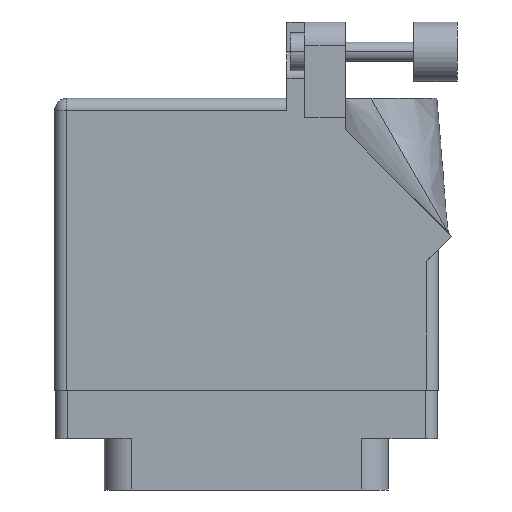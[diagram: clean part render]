
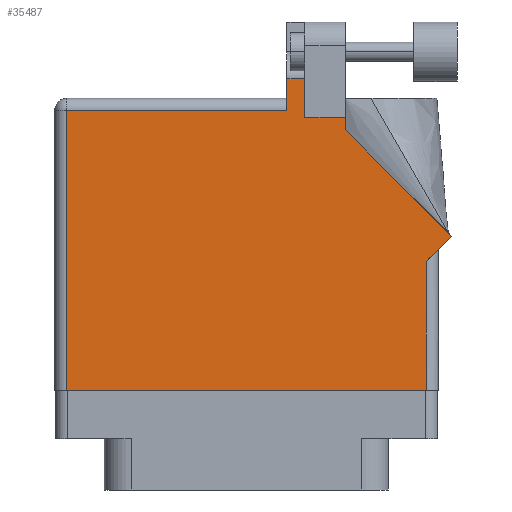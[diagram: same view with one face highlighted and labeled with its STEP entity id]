
A CAD part, front view. The second image highlights one B-rep face of the part: STEP entity #35487.
In plain terms, the highlighted face is planar.
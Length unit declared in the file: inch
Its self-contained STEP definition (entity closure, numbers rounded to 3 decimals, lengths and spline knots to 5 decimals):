
#379 = VECTOR ( 'NONE', #23614, 39.37008 ) ;
#653 = VECTOR ( 'NONE', #24554, 39.37008 ) ;
#1255 = EDGE_CURVE ( 'NONE', #32799, #14136, #2132, .T. ) ;
#1619 = ORIENTED_EDGE ( 'NONE', *, *, #6178, .T. ) ;
#2132 = LINE ( 'NONE', #20921, #379 ) ;
#3092 = ORIENTED_EDGE ( 'NONE', *, *, #34609, .T. ) ;
#3384 = VERTEX_POINT ( 'NONE', #27322 ) ;
#3631 = VECTOR ( 'NONE', #16122, 39.37008 ) ;
#3698 = AXIS2_PLACEMENT_3D ( 'NONE', #28325, #28918, #32117 ) ;
#4197 = CARTESIAN_POINT ( 'NONE',  ( 0.306, 1.33, 0.455 ) ) ;
#4200 = LINE ( 'NONE', #22063, #33316 ) ;
#4429 = LINE ( 'NONE', #13375, #14575 ) ;
#5125 = CARTESIAN_POINT ( 'NONE',  ( 0.63677, 1.5315, 0.455 ) ) ;
#6178 = EDGE_CURVE ( 'NONE', #30503, #13214, #19318, .T. ) ;
#6745 = ORIENTED_EDGE ( 'NONE', *, *, #1255, .T. ) ;
#7783 = DIRECTION ( 'NONE',  ( -0.707, 0.707, 0. ) ) ;
#8023 = CARTESIAN_POINT ( 'NONE',  ( 0.519, 1.26442, 0.455 ) ) ;
#8145 = LINE ( 'NONE', #21734, #653 ) ;
#8902 = ORIENTED_EDGE ( 'NONE', *, *, #35794, .T. ) ;
#9050 = CARTESIAN_POINT ( 'NONE',  ( -0.943, -0.1, 0.455 ) ) ;
#9063 = LINE ( 'NONE', #27660, #13047 ) ;
#9408 = CARTESIAN_POINT ( 'NONE',  ( 1.07571, 0.70771, 0.455 ) ) ;
#10152 = EDGE_CURVE ( 'NONE', #3384, #30298, #11597, .T. ) ;
#10605 = CARTESIAN_POINT ( 'NONE',  ( 0.519, 1.26442, 0.455 ) ) ;
#11462 = VECTOR ( 'NONE', #28181, 39.37008 ) ;
#11514 = ORIENTED_EDGE ( 'NONE', *, *, #27716, .T. ) ;
#11526 = VECTOR ( 'NONE', #19142, 39.37008 ) ;
#11597 = LINE ( 'NONE', #21714, #3631 ) ;
#12305 = VERTEX_POINT ( 'NONE', #13595 ) ;
#12872 = DIRECTION ( 'NONE',  ( 0., -1., 0. ) ) ;
#13047 = VECTOR ( 'NONE', #36374, 39.37008 ) ;
#13214 = VERTEX_POINT ( 'NONE', #8023 ) ;
#13375 = CARTESIAN_POINT ( 'NONE',  ( 1.005, 0.637, 0.455 ) ) ;
#13595 = CARTESIAN_POINT ( 'NONE',  ( 0.306, 1.5315, 0.455 ) ) ;
#14136 = VERTEX_POINT ( 'NONE', #34567 ) ;
#14575 = VECTOR ( 'NONE', #16202, 39.37008 ) ;
#14592 = VECTOR ( 'NONE', #23226, 39.37008 ) ;
#15504 = LINE ( 'NONE', #10605, #11526 ) ;
#15553 = ORIENTED_EDGE ( 'NONE', *, *, #17879, .T. ) ;
#16122 = DIRECTION ( 'NONE',  ( 0., -1., 0. ) ) ;
#16136 = VECTOR ( 'NONE', #12872, 39.37008 ) ;
#16202 = DIRECTION ( 'NONE',  ( 0.707, 0.707, 0. ) ) ;
#16537 = VERTEX_POINT ( 'NONE', #33179 ) ;
#17108 = VECTOR ( 'NONE', #7783, 39.37008 ) ;
#17392 = VERTEX_POINT ( 'NONE', #18812 ) ;
#17879 = EDGE_CURVE ( 'NONE', #33419, #17392, #23655, .T. ) ;
#18084 = FACE_OUTER_BOUND ( 'NONE', #23627, .T. ) ;
#18812 = CARTESIAN_POINT ( 'NONE',  ( 0.212, 1.368, 0.455 ) ) ;
#19142 = DIRECTION ( 'NONE',  ( 0., 1., 0. ) ) ;
#19318 = LINE ( 'NONE', #36235, #17108 ) ;
#19825 = PLANE ( 'NONE',  #3698 ) ;
#20921 = CARTESIAN_POINT ( 'NONE',  ( 0.943, 0.637, 0.455 ) ) ;
#20997 = VERTEX_POINT ( 'NONE', #4197 ) ;
#21714 = CARTESIAN_POINT ( 'NONE',  ( -0.943, -0.1, 0.455 ) ) ;
#21734 = CARTESIAN_POINT ( 'NONE',  ( -1.005, -0.1, 0.455 ) ) ;
#22063 = CARTESIAN_POINT ( 'NONE',  ( 0.519, 1.33, 0.455 ) ) ;
#22967 = LINE ( 'NONE', #23095, #14592 ) ;
#23095 = CARTESIAN_POINT ( 'NONE',  ( 0.306, 1.33, 0.455 ) ) ;
#23226 = DIRECTION ( 'NONE',  ( 0., 1., 0. ) ) ;
#23614 = DIRECTION ( 'NONE',  ( 0., 1., 0. ) ) ;
#23627 = EDGE_LOOP ( 'NONE', ( #33123, #8902, #15553, #27312, #23972, #25921, #6745, #32925, #1619, #3092, #11514 ) ) ;
#23655 = LINE ( 'NONE', #29771, #16136 ) ;
#23972 = ORIENTED_EDGE ( 'NONE', *, *, #10152, .T. ) ;
#24507 = EDGE_CURVE ( 'NONE', #14136, #30503, #4429, .T. ) ;
#24554 = DIRECTION ( 'NONE',  ( 1., 0., 0. ) ) ;
#25921 = ORIENTED_EDGE ( 'NONE', *, *, #31208, .T. ) ;
#27004 = EDGE_CURVE ( 'NONE', #17392, #3384, #9063, .T. ) ;
#27312 = ORIENTED_EDGE ( 'NONE', *, *, #27004, .T. ) ;
#27322 = CARTESIAN_POINT ( 'NONE',  ( -0.943, 1.368, 0.455 ) ) ;
#27660 = CARTESIAN_POINT ( 'NONE',  ( -1.005, 1.368, 0.455 ) ) ;
#27716 = EDGE_CURVE ( 'NONE', #16537, #20997, #4200, .T. ) ;
#28181 = DIRECTION ( 'NONE',  ( -1., 0., 0. ) ) ;
#28325 = CARTESIAN_POINT ( 'NONE',  ( -1.005, 1.43, 0.455 ) ) ;
#28918 = DIRECTION ( 'NONE',  ( 0., 0., -1. ) ) ;
#29113 = LINE ( 'NONE', #5125, #11462 ) ;
#29771 = CARTESIAN_POINT ( 'NONE',  ( 0.212, 1.43, 0.455 ) ) ;
#29903 = CARTESIAN_POINT ( 'NONE',  ( 0.943, -0.1, 0.455 ) ) ;
#30114 = CARTESIAN_POINT ( 'NONE',  ( 0.212, 1.5315, 0.455 ) ) ;
#30298 = VERTEX_POINT ( 'NONE', #9050 ) ;
#30438 = DIRECTION ( 'NONE',  ( -1., 0., 0. ) ) ;
#30503 = VERTEX_POINT ( 'NONE', #9408 ) ;
#31208 = EDGE_CURVE ( 'NONE', #30298, #32799, #8145, .T. ) ;
#32117 = DIRECTION ( 'NONE',  ( -1., 0., 0. ) ) ;
#32799 = VERTEX_POINT ( 'NONE', #29903 ) ;
#32925 = ORIENTED_EDGE ( 'NONE', *, *, #24507, .T. ) ;
#33123 = ORIENTED_EDGE ( 'NONE', *, *, #34312, .T. ) ;
#33179 = CARTESIAN_POINT ( 'NONE',  ( 0.519, 1.33, 0.455 ) ) ;
#33316 = VECTOR ( 'NONE', #30438, 39.37008 ) ;
#33419 = VERTEX_POINT ( 'NONE', #30114 ) ;
#34312 = EDGE_CURVE ( 'NONE', #20997, #12305, #22967, .T. ) ;
#34567 = CARTESIAN_POINT ( 'NONE',  ( 0.943, 0.575, 0.455 ) ) ;
#34609 = EDGE_CURVE ( 'NONE', #13214, #16537, #15504, .T. ) ;
#35487 = ADVANCED_FACE ( 'NONE', ( #18084 ), #19825, .F. ) ;
#35794 = EDGE_CURVE ( 'NONE', #12305, #33419, #29113, .T. ) ;
#36235 = CARTESIAN_POINT ( 'NONE',  ( 1.07571, 0.70771, 0.455 ) ) ;
#36374 = DIRECTION ( 'NONE',  ( -1., 0., 0. ) ) ;
